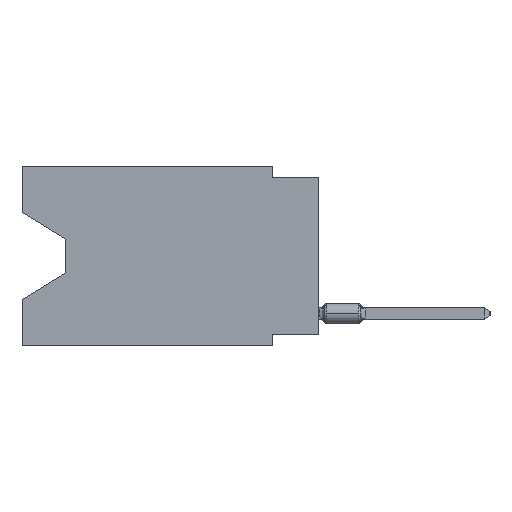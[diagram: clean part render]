
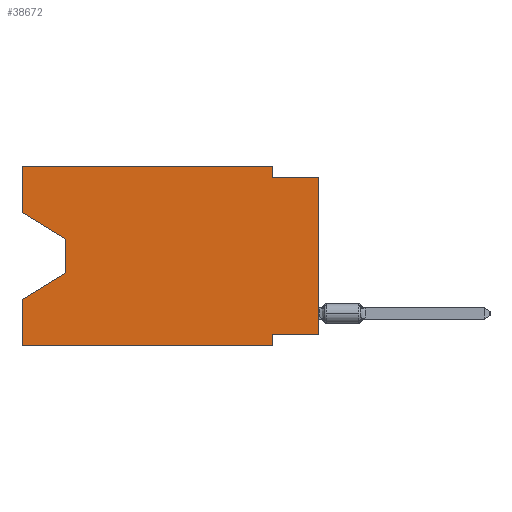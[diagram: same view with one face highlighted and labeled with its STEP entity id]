
A CAD part, left-side view. The second image highlights one B-rep face of the part: STEP entity #38672.
In plain terms, the highlighted planar face has unit normal (-1, 0, 0).
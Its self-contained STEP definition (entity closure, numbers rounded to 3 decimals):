
#9 = CARTESIAN_POINT ( 'NONE',  ( 0., 13.97, -4.013 ) ) ;
#436 = LINE ( 'NONE', #3463, #34063 ) ;
#1092 = LINE ( 'NONE', #23545, #40051 ) ;
#3163 = ORIENTED_EDGE ( 'NONE', *, *, #29517, .F. ) ;
#3388 = DIRECTION ( 'NONE',  ( 0., 0., 1. ) ) ;
#3463 = CARTESIAN_POINT ( 'NONE',  ( 0., 2.54, -9.906 ) ) ;
#3791 = VECTOR ( 'NONE', #9690, 1000. ) ;
#4539 = DIRECTION ( 'NONE',  ( 0., -0.855, -0.519 ) ) ;
#5410 = EDGE_CURVE ( 'NONE', #10311, #30797, #48103, .T. ) ;
#6729 = CARTESIAN_POINT ( 'NONE',  ( 0., 16.383, -2.546 ) ) ;
#7321 = CARTESIAN_POINT ( 'NONE',  ( 0., 13.97, -5.893 ) ) ;
#8591 = CARTESIAN_POINT ( 'NONE',  ( 0., 16.383, -9.906 ) ) ;
#8920 = ORIENTED_EDGE ( 'NONE', *, *, #43894, .F. ) ;
#9690 = DIRECTION ( 'NONE',  ( 0., 0., 1. ) ) ;
#10194 = CARTESIAN_POINT ( 'NONE',  ( 0., 0., -0.635 ) ) ;
#10308 = CARTESIAN_POINT ( 'NONE',  ( 0., 16.383, 0. ) ) ;
#10311 = VERTEX_POINT ( 'NONE', #6729 ) ;
#11494 = VECTOR ( 'NONE', #30105, 1000. ) ;
#11946 = LINE ( 'NONE', #14998, #23186 ) ;
#12589 = EDGE_CURVE ( 'NONE', #27696, #37548, #22298, .T. ) ;
#13266 = ORIENTED_EDGE ( 'NONE', *, *, #38951, .T. ) ;
#13949 = EDGE_LOOP ( 'NONE', ( #34874, #23181, #23322, #22098, #13266, #3163, #43671, #30805, #49117, #8920, #33097, #32097 ) ) ;
#14744 = LINE ( 'NONE', #10194, #11494 ) ;
#14998 = CARTESIAN_POINT ( 'NONE',  ( 0., 13.97, -4.013 ) ) ;
#15707 = VECTOR ( 'NONE', #4539, 1000. ) ;
#15713 = DIRECTION ( 'NONE',  ( 0., 0., -1. ) ) ;
#20811 = CARTESIAN_POINT ( 'NONE',  ( 0., 16.383, 0. ) ) ;
#21434 = FACE_OUTER_BOUND ( 'NONE', #13949, .T. ) ;
#21676 = PLANE ( 'NONE',  #35421 ) ;
#21809 = VECTOR ( 'NONE', #43473, 1000. ) ;
#22098 = ORIENTED_EDGE ( 'NONE', *, *, #43622, .F. ) ;
#22298 = LINE ( 'NONE', #26823, #46372 ) ;
#23181 = ORIENTED_EDGE ( 'NONE', *, *, #34010, .T. ) ;
#23186 = VECTOR ( 'NONE', #27334, 1000. ) ;
#23322 = ORIENTED_EDGE ( 'NONE', *, *, #48830, .T. ) ;
#23545 = CARTESIAN_POINT ( 'NONE',  ( 0., 2.54, 0. ) ) ;
#23608 = EDGE_CURVE ( 'NONE', #38508, #37548, #14744, .T. ) ;
#24152 = EDGE_CURVE ( 'NONE', #30797, #39528, #32521, .T. ) ;
#25470 = DIRECTION ( 'NONE',  ( 1., 0., 0. ) ) ;
#25548 = LINE ( 'NONE', #36606, #36904 ) ;
#25794 = DIRECTION ( 'NONE',  ( 0., 1., 0. ) ) ;
#26304 = CARTESIAN_POINT ( 'NONE',  ( 0., 16.383, -7.36 ) ) ;
#26633 = CARTESIAN_POINT ( 'NONE',  ( 0., 0., -0.635 ) ) ;
#26823 = CARTESIAN_POINT ( 'NONE',  ( 0., 0., 0. ) ) ;
#27334 = DIRECTION ( 'NONE',  ( 0., 0., -1. ) ) ;
#27696 = VERTEX_POINT ( 'NONE', #35901 ) ;
#29160 = CARTESIAN_POINT ( 'NONE',  ( 0., 2.54, -9.271 ) ) ;
#29293 = CARTESIAN_POINT ( 'NONE',  ( 0., 2.54, 0. ) ) ;
#29517 = EDGE_CURVE ( 'NONE', #40759, #46118, #436, .T. ) ;
#29535 = VERTEX_POINT ( 'NONE', #34681 ) ;
#29901 = VECTOR ( 'NONE', #38815, 1000. ) ;
#30105 = DIRECTION ( 'NONE',  ( 0., -1., 0. ) ) ;
#30797 = VERTEX_POINT ( 'NONE', #42499 ) ;
#30805 = ORIENTED_EDGE ( 'NONE', *, *, #12589, .T. ) ;
#31246 = CARTESIAN_POINT ( 'NONE',  ( 0., 16.383, -2.546 ) ) ;
#32097 = ORIENTED_EDGE ( 'NONE', *, *, #5410, .F. ) ;
#32129 = LINE ( 'NONE', #20811, #3791 ) ;
#32521 = LINE ( 'NONE', #47888, #34048 ) ;
#33097 = ORIENTED_EDGE ( 'NONE', *, *, #24152, .F. ) ;
#33309 = VERTEX_POINT ( 'NONE', #8591 ) ;
#34010 = EDGE_CURVE ( 'NONE', #45571, #29535, #11946, .T. ) ;
#34048 = VECTOR ( 'NONE', #47638, 1000. ) ;
#34063 = VECTOR ( 'NONE', #38230, 1000. ) ;
#34681 = CARTESIAN_POINT ( 'NONE',  ( 0., 13.97, -5.893 ) ) ;
#34874 = ORIENTED_EDGE ( 'NONE', *, *, #41412, .T. ) ;
#35421 = AXIS2_PLACEMENT_3D ( 'NONE', #10308, #25470, #36769 ) ;
#35901 = CARTESIAN_POINT ( 'NONE',  ( 0., 0., -9.271 ) ) ;
#36606 = CARTESIAN_POINT ( 'NONE',  ( 0., 0., -9.271 ) ) ;
#36769 = DIRECTION ( 'NONE',  ( 0., 0., -1. ) ) ;
#36868 = CARTESIAN_POINT ( 'NONE',  ( 0., 2.54, -9.906 ) ) ;
#36904 = VECTOR ( 'NONE', #25794, 1000. ) ;
#37548 = VERTEX_POINT ( 'NONE', #26633 ) ;
#38230 = DIRECTION ( 'NONE',  ( 0., 0., -1. ) ) ;
#38508 = VERTEX_POINT ( 'NONE', #46878 ) ;
#38672 = ADVANCED_FACE ( 'NONE', ( #21434 ), #21676, .F. ) ;
#38815 = DIRECTION ( 'NONE',  ( 0., 0.855, -0.519 ) ) ;
#38951 = EDGE_CURVE ( 'NONE', #33309, #46118, #47996, .T. ) ;
#39056 = LINE ( 'NONE', #31246, #15707 ) ;
#39528 = VERTEX_POINT ( 'NONE', #29293 ) ;
#39558 = DIRECTION ( 'NONE',  ( 0., 0., 1. ) ) ;
#40051 = VECTOR ( 'NONE', #15713, 1000. ) ;
#40444 = CARTESIAN_POINT ( 'NONE',  ( 0., 16.383, -9.906 ) ) ;
#40759 = VERTEX_POINT ( 'NONE', #29160 ) ;
#40975 = VECTOR ( 'NONE', #39558, 1000. ) ;
#41324 = VERTEX_POINT ( 'NONE', #26304 ) ;
#41412 = EDGE_CURVE ( 'NONE', #10311, #45571, #39056, .T. ) ;
#42499 = CARTESIAN_POINT ( 'NONE',  ( 0., 16.383, 0. ) ) ;
#42579 = LINE ( 'NONE', #7321, #29901 ) ;
#43473 = DIRECTION ( 'NONE',  ( 0., -1., 0. ) ) ;
#43622 = EDGE_CURVE ( 'NONE', #33309, #41324, #32129, .T. ) ;
#43671 = ORIENTED_EDGE ( 'NONE', *, *, #45037, .F. ) ;
#43894 = EDGE_CURVE ( 'NONE', #39528, #38508, #1092, .T. ) ;
#45037 = EDGE_CURVE ( 'NONE', #27696, #40759, #25548, .T. ) ;
#45571 = VERTEX_POINT ( 'NONE', #9 ) ;
#46118 = VERTEX_POINT ( 'NONE', #36868 ) ;
#46372 = VECTOR ( 'NONE', #3388, 1000. ) ;
#46878 = CARTESIAN_POINT ( 'NONE',  ( 0., 2.54, -0.635 ) ) ;
#47607 = CARTESIAN_POINT ( 'NONE',  ( 0., 16.383, 0. ) ) ;
#47638 = DIRECTION ( 'NONE',  ( 0., -1., 0. ) ) ;
#47888 = CARTESIAN_POINT ( 'NONE',  ( 0., 16.383, 0. ) ) ;
#47996 = LINE ( 'NONE', #40444, #21809 ) ;
#48103 = LINE ( 'NONE', #47607, #40975 ) ;
#48830 = EDGE_CURVE ( 'NONE', #29535, #41324, #42579, .T. ) ;
#49117 = ORIENTED_EDGE ( 'NONE', *, *, #23608, .F. ) ;
